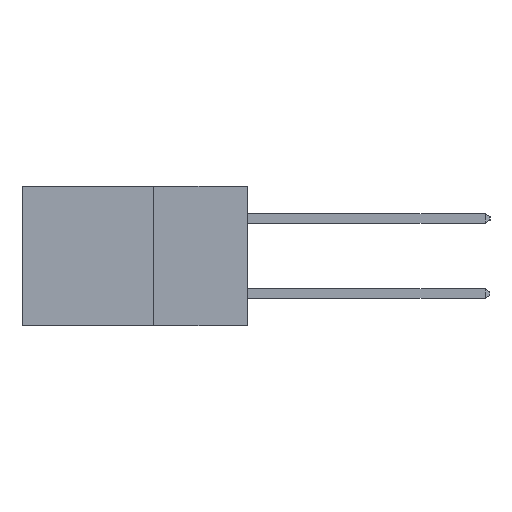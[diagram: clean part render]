
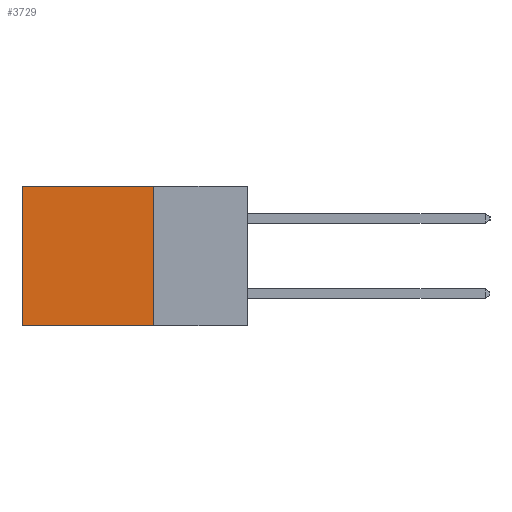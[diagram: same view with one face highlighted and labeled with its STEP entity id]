
A CAD part, left-side view. The second image highlights one B-rep face of the part: STEP entity #3729.
In plain terms, the highlighted planar face has unit normal (-1, 0, 0).
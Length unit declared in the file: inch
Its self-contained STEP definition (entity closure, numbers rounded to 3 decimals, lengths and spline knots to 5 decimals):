
#1682 = FACE_OUTER_BOUND ( 'NONE', #11918, .T. ) ;
#2520 = LINE ( 'NONE', #7417, #16009 ) ;
#2623 = EDGE_CURVE ( 'NONE', #15321, #16832, #10484, .T. ) ;
#2686 = EDGE_CURVE ( 'NONE', #12332, #10540, #6238, .T. ) ;
#3729 = ADVANCED_FACE ( 'NONE', ( #1682 ), #7767, .F. ) ;
#4761 = VECTOR ( 'NONE', #5830, 39.37008 ) ;
#5830 = DIRECTION ( 'NONE',  ( 0., 0., -1. ) ) ;
#6238 = LINE ( 'NONE', #14958, #16095 ) ;
#7030 = CARTESIAN_POINT ( 'NONE',  ( 0.298, 0.25, -0.37 ) ) ;
#7417 = CARTESIAN_POINT ( 'NONE',  ( 0.298, 0.6, 0. ) ) ;
#7432 = CARTESIAN_POINT ( 'NONE',  ( 0.298, 0.25, 0. ) ) ;
#7767 = PLANE ( 'NONE',  #13208 ) ;
#8019 = CARTESIAN_POINT ( 'NONE',  ( 0.298, 0.25, 0. ) ) ;
#8448 = CARTESIAN_POINT ( 'NONE',  ( 0.298, 0.6, -0.37 ) ) ;
#8710 = DIRECTION ( 'NONE',  ( 0., 0., -1. ) ) ;
#8913 = DIRECTION ( 'NONE',  ( 0., 0., -1. ) ) ;
#8983 = DIRECTION ( 'NONE',  ( 1., 0., 0. ) ) ;
#9077 = ORIENTED_EDGE ( 'NONE', *, *, #2623, .F. ) ;
#10484 = LINE ( 'NONE', #11109, #16887 ) ;
#10540 = VERTEX_POINT ( 'NONE', #13437 ) ;
#11109 = CARTESIAN_POINT ( 'NONE',  ( 0.298, 0.25, -0.37 ) ) ;
#11278 = ORIENTED_EDGE ( 'NONE', *, *, #16306, .F. ) ;
#11918 = EDGE_LOOP ( 'NONE', ( #12542, #9077, #11278, #12477 ) ) ;
#12021 = DIRECTION ( 'NONE',  ( 0., 1., 0. ) ) ;
#12275 = CARTESIAN_POINT ( 'NONE',  ( 0.298, 0.25, 0. ) ) ;
#12332 = VERTEX_POINT ( 'NONE', #8019 ) ;
#12477 = ORIENTED_EDGE ( 'NONE', *, *, #2686, .T. ) ;
#12542 = ORIENTED_EDGE ( 'NONE', *, *, #13695, .T. ) ;
#13208 = AXIS2_PLACEMENT_3D ( 'NONE', #7432, #8983, #8913 ) ;
#13437 = CARTESIAN_POINT ( 'NONE',  ( 0.298, 0.6, 0. ) ) ;
#13695 = EDGE_CURVE ( 'NONE', #10540, #16832, #2520, .T. ) ;
#14958 = CARTESIAN_POINT ( 'NONE',  ( 0.298, 0.25, 0. ) ) ;
#15116 = LINE ( 'NONE', #12275, #4761 ) ;
#15321 = VERTEX_POINT ( 'NONE', #7030 ) ;
#16009 = VECTOR ( 'NONE', #8710, 39.37008 ) ;
#16095 = VECTOR ( 'NONE', #16686, 39.37008 ) ;
#16306 = EDGE_CURVE ( 'NONE', #12332, #15321, #15116, .T. ) ;
#16686 = DIRECTION ( 'NONE',  ( 0., 1., 0. ) ) ;
#16832 = VERTEX_POINT ( 'NONE', #8448 ) ;
#16887 = VECTOR ( 'NONE', #12021, 39.37008 ) ;
